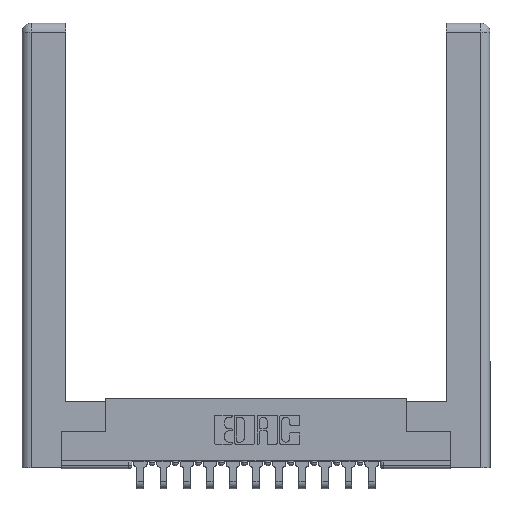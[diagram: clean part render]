
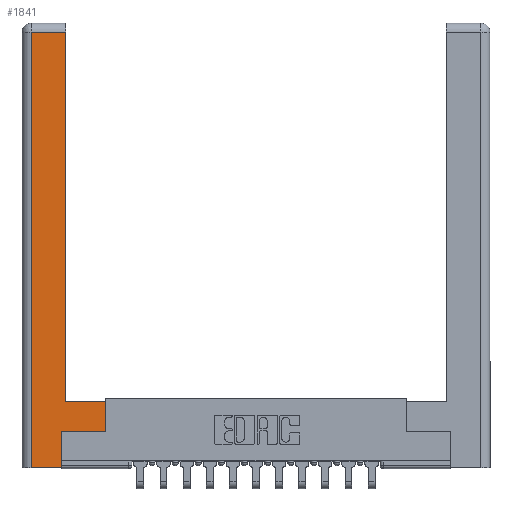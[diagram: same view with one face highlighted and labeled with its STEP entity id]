
A CAD part, top view. The second image highlights one B-rep face of the part: STEP entity #1841.
In plain terms, the highlighted planar face has unit normal (0, 0, 1).
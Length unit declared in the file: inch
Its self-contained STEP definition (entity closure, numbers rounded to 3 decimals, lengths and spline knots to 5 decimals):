
#40 = EDGE_LOOP ( 'NONE', ( #7702, #12084, #4254, #3910, #5101, #14911, #4327, #9287 ) ) ;
#58 = VECTOR ( 'NONE', #284, 39.37008 ) ;
#149 = DIRECTION ( 'NONE',  ( -1., 0., 0. ) ) ;
#199 = VECTOR ( 'NONE', #15463, 39.37008 ) ;
#208 = VERTEX_POINT ( 'NONE', #3844 ) ;
#229 = EDGE_CURVE ( 'NONE', #11876, #8771, #9797, .T. ) ;
#284 = DIRECTION ( 'NONE',  ( -1., 0., 0. ) ) ;
#330 = EDGE_CURVE ( 'NONE', #208, #7740, #1879, .T. ) ;
#507 = CARTESIAN_POINT ( 'NONE',  ( 0.295, 3., 0. ) ) ;
#1086 = VERTEX_POINT ( 'NONE', #5582 ) ;
#1841 = ADVANCED_FACE ( 'NONE', ( #7583 ), #14761, .F. ) ;
#1879 = LINE ( 'NONE', #15042, #10753 ) ;
#2220 = CARTESIAN_POINT ( 'NONE',  ( 0.295, 0.45, 0. ) ) ;
#2313 = LINE ( 'NONE', #14467, #13892 ) ;
#3093 = CARTESIAN_POINT ( 'NONE',  ( 0.265, 0.245, 0. ) ) ;
#3844 = CARTESIAN_POINT ( 'NONE',  ( 0.0615, 0., 0. ) ) ;
#3910 = ORIENTED_EDGE ( 'NONE', *, *, #330, .T. ) ;
#4254 = ORIENTED_EDGE ( 'NONE', *, *, #11013, .T. ) ;
#4327 = ORIENTED_EDGE ( 'NONE', *, *, #14428, .T. ) ;
#4647 = EDGE_CURVE ( 'NONE', #7740, #8695, #2313, .T. ) ;
#5101 = ORIENTED_EDGE ( 'NONE', *, *, #4647, .T. ) ;
#5127 = CARTESIAN_POINT ( 'NONE',  ( 0., 0., 0. ) ) ;
#5582 = CARTESIAN_POINT ( 'NONE',  ( 0.295, 2.94, 0. ) ) ;
#5948 = DIRECTION ( 'NONE',  ( 0., 1., 0. ) ) ;
#6204 = LINE ( 'NONE', #11718, #199 ) ;
#7085 = CARTESIAN_POINT ( 'NONE',  ( 0.565, 0.45, 0. ) ) ;
#7205 = DIRECTION ( 'NONE',  ( 1., 0., 0. ) ) ;
#7279 = VECTOR ( 'NONE', #13670, 39.37008 ) ;
#7352 = CARTESIAN_POINT ( 'NONE',  ( 0.265, 0., 0. ) ) ;
#7473 = EDGE_CURVE ( 'NONE', #8695, #14278, #6204, .T. ) ;
#7583 = FACE_OUTER_BOUND ( 'NONE', #40, .T. ) ;
#7655 = CARTESIAN_POINT ( 'NONE',  ( 0.0615, 2.94, 0. ) ) ;
#7702 = ORIENTED_EDGE ( 'NONE', *, *, #11657, .T. ) ;
#7740 = VERTEX_POINT ( 'NONE', #7352 ) ;
#7841 = DIRECTION ( 'NONE',  ( 0., 1., 0. ) ) ;
#8409 = VECTOR ( 'NONE', #13097, 39.37008 ) ;
#8695 = VERTEX_POINT ( 'NONE', #3093 ) ;
#8696 = CARTESIAN_POINT ( 'NONE',  ( 0.295, 0.45, 0. ) ) ;
#8771 = VERTEX_POINT ( 'NONE', #2220 ) ;
#9287 = ORIENTED_EDGE ( 'NONE', *, *, #229, .T. ) ;
#9797 = LINE ( 'NONE', #8696, #7279 ) ;
#10682 = LINE ( 'NONE', #7655, #58 ) ;
#10699 = VECTOR ( 'NONE', #5948, 39.37008 ) ;
#10753 = VECTOR ( 'NONE', #7205, 39.37008 ) ;
#11013 = EDGE_CURVE ( 'NONE', #11836, #208, #11300, .T. ) ;
#11284 = LINE ( 'NONE', #13338, #10699 ) ;
#11300 = LINE ( 'NONE', #12992, #8409 ) ;
#11657 = EDGE_CURVE ( 'NONE', #8771, #1086, #12244, .T. ) ;
#11718 = CARTESIAN_POINT ( 'NONE',  ( 0.565, 0.245, 0. ) ) ;
#11762 = CARTESIAN_POINT ( 'NONE',  ( 0.0615, 2.94, 0. ) ) ;
#11836 = VERTEX_POINT ( 'NONE', #11762 ) ;
#11876 = VERTEX_POINT ( 'NONE', #7085 ) ;
#12084 = ORIENTED_EDGE ( 'NONE', *, *, #12162, .T. ) ;
#12162 = EDGE_CURVE ( 'NONE', #1086, #11836, #10682, .T. ) ;
#12244 = LINE ( 'NONE', #507, #14744 ) ;
#12690 = CARTESIAN_POINT ( 'NONE',  ( 0.565, 0.245, 0. ) ) ;
#12992 = CARTESIAN_POINT ( 'NONE',  ( 0.0615, 0., 0. ) ) ;
#13097 = DIRECTION ( 'NONE',  ( 0., -1., 0. ) ) ;
#13338 = CARTESIAN_POINT ( 'NONE',  ( 0.565, 0.45, 0. ) ) ;
#13670 = DIRECTION ( 'NONE',  ( -1., 0., 0. ) ) ;
#13892 = VECTOR ( 'NONE', #15821, 39.37008 ) ;
#14278 = VERTEX_POINT ( 'NONE', #12690 ) ;
#14428 = EDGE_CURVE ( 'NONE', #14278, #11876, #11284, .T. ) ;
#14467 = CARTESIAN_POINT ( 'NONE',  ( 0.265, 0.245, 0. ) ) ;
#14580 = AXIS2_PLACEMENT_3D ( 'NONE', #5127, #14927, #149 ) ;
#14744 = VECTOR ( 'NONE', #7841, 39.37008 ) ;
#14761 = PLANE ( 'NONE',  #14580 ) ;
#14911 = ORIENTED_EDGE ( 'NONE', *, *, #7473, .T. ) ;
#14927 = DIRECTION ( 'NONE',  ( 0., 0., -1. ) ) ;
#15042 = CARTESIAN_POINT ( 'NONE',  ( 0.265, 0., 0. ) ) ;
#15463 = DIRECTION ( 'NONE',  ( 1., 0., 0. ) ) ;
#15821 = DIRECTION ( 'NONE',  ( 0., 1., 0. ) ) ;
